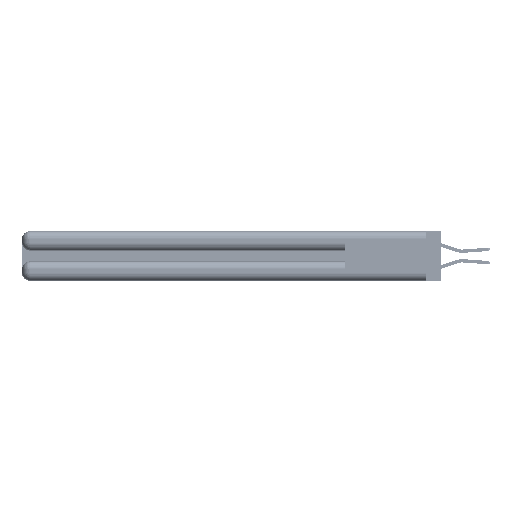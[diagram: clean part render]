
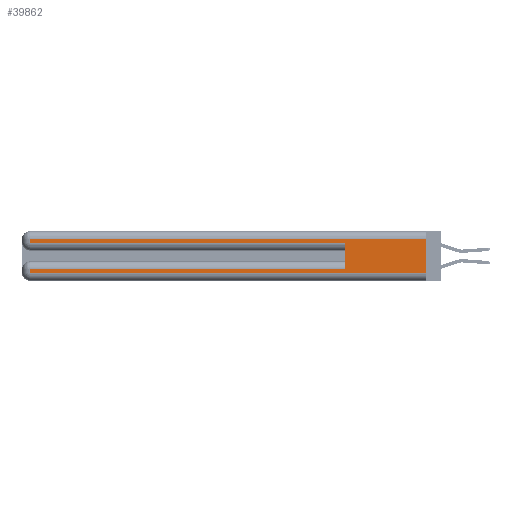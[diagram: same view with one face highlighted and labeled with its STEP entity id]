
A CAD part, left-side view. The second image highlights one B-rep face of the part: STEP entity #39862.
In plain terms, the highlighted planar face has unit normal (-1, 0, 0).
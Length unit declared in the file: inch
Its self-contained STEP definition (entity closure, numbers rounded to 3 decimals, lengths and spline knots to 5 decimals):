
#19 = EDGE_LOOP ( 'NONE', ( #41793, #40045, #23522, #11008, #38077, #45327, #18876, #37443 ) ) ;
#169 = LINE ( 'NONE', #45112, #32521 ) ;
#388 = LINE ( 'NONE', #1569, #31431 ) ;
#1320 = VERTEX_POINT ( 'NONE', #47168 ) ;
#1569 = CARTESIAN_POINT ( 'NONE',  ( 0., 2.94, 0.37 ) ) ;
#1657 = DIRECTION ( 'NONE',  ( 0., 1., 0. ) ) ;
#2510 = CARTESIAN_POINT ( 'NONE',  ( 0., 2.94, 0.285 ) ) ;
#3579 = DIRECTION ( 'NONE',  ( 0., -1., 0. ) ) ;
#3633 = VERTEX_POINT ( 'NONE', #2510 ) ;
#5239 = VECTOR ( 'NONE', #3579, 39.37008 ) ;
#7602 = EDGE_CURVE ( 'NONE', #53940, #32389, #27688, .T. ) ;
#9394 = VECTOR ( 'NONE', #11906, 39.37008 ) ;
#11008 = ORIENTED_EDGE ( 'NONE', *, *, #33853, .T. ) ;
#11906 = DIRECTION ( 'NONE',  ( 0., 0., -1. ) ) ;
#12289 = PLANE ( 'NONE',  #41808 ) ;
#12951 = VERTEX_POINT ( 'NONE', #17623 ) ;
#13339 = CARTESIAN_POINT ( 'NONE',  ( 0., 0., 0.31 ) ) ;
#14971 = CARTESIAN_POINT ( 'NONE',  ( 0., 2.94, 0.31 ) ) ;
#14999 = EDGE_CURVE ( 'NONE', #12951, #39298, #43915, .T. ) ;
#15232 = EDGE_CURVE ( 'NONE', #39298, #53940, #48528, .T. ) ;
#16108 = CARTESIAN_POINT ( 'NONE',  ( 0., 0., 0.06 ) ) ;
#16532 = DIRECTION ( 'NONE',  ( 0., 0., -1. ) ) ;
#17623 = CARTESIAN_POINT ( 'NONE',  ( 0., 0.6, 0.085 ) ) ;
#18876 = ORIENTED_EDGE ( 'NONE', *, *, #15232, .T. ) ;
#21177 = CARTESIAN_POINT ( 'NONE',  ( 0., 0., 0.285 ) ) ;
#22889 = VERTEX_POINT ( 'NONE', #14971 ) ;
#23522 = ORIENTED_EDGE ( 'NONE', *, *, #53543, .T. ) ;
#24090 = DIRECTION ( 'NONE',  ( 0., 0., 1. ) ) ;
#24124 = VECTOR ( 'NONE', #1657, 39.37008 ) ;
#25426 = DIRECTION ( 'NONE',  ( 0., -1., 0. ) ) ;
#26855 = DIRECTION ( 'NONE',  ( 0., 0., -1. ) ) ;
#26941 = CARTESIAN_POINT ( 'NONE',  ( 0., 0., 0.085 ) ) ;
#27688 = LINE ( 'NONE', #16108, #5239 ) ;
#30263 = FACE_OUTER_BOUND ( 'NONE', #19, .T. ) ;
#30709 = EDGE_CURVE ( 'NONE', #12951, #41494, #169, .T. ) ;
#31431 = VECTOR ( 'NONE', #26855, 39.37008 ) ;
#32170 = VECTOR ( 'NONE', #25426, 39.37008 ) ;
#32389 = VERTEX_POINT ( 'NONE', #45517 ) ;
#32521 = VECTOR ( 'NONE', #24090, 39.37008 ) ;
#32956 = CARTESIAN_POINT ( 'NONE',  ( 0., 0., 0.37 ) ) ;
#33336 = VECTOR ( 'NONE', #49042, 39.37008 ) ;
#33473 = LINE ( 'NONE', #21177, #32170 ) ;
#33578 = CARTESIAN_POINT ( 'NONE',  ( 0., 2.94, 0.085 ) ) ;
#33853 = EDGE_CURVE ( 'NONE', #3633, #41494, #33473, .T. ) ;
#37443 = ORIENTED_EDGE ( 'NONE', *, *, #7602, .T. ) ;
#37592 = CARTESIAN_POINT ( 'NONE',  ( 0., 0., 0.37 ) ) ;
#38077 = ORIENTED_EDGE ( 'NONE', *, *, #30709, .F. ) ;
#38658 = DIRECTION ( 'NONE',  ( 0., 1., 0. ) ) ;
#39298 = VERTEX_POINT ( 'NONE', #33578 ) ;
#39862 = ADVANCED_FACE ( 'NONE', ( #30263 ), #12289, .F. ) ;
#40045 = ORIENTED_EDGE ( 'NONE', *, *, #40346, .T. ) ;
#40346 = EDGE_CURVE ( 'NONE', #1320, #22889, #41411, .T. ) ;
#41411 = LINE ( 'NONE', #13339, #51311 ) ;
#41494 = VERTEX_POINT ( 'NONE', #54573 ) ;
#41793 = ORIENTED_EDGE ( 'NONE', *, *, #48043, .F. ) ;
#41808 = AXIS2_PLACEMENT_3D ( 'NONE', #37592, #41818, #16532 ) ;
#41818 = DIRECTION ( 'NONE',  ( 1., 0., 0. ) ) ;
#43043 = LINE ( 'NONE', #32956, #9394 ) ;
#43915 = LINE ( 'NONE', #26941, #24124 ) ;
#45112 = CARTESIAN_POINT ( 'NONE',  ( 0., 0.6, 0.145 ) ) ;
#45327 = ORIENTED_EDGE ( 'NONE', *, *, #14999, .T. ) ;
#45517 = CARTESIAN_POINT ( 'NONE',  ( 0., 0., 0.06 ) ) ;
#47168 = CARTESIAN_POINT ( 'NONE',  ( 0., 0., 0.31 ) ) ;
#48043 = EDGE_CURVE ( 'NONE', #1320, #32389, #43043, .T. ) ;
#48528 = LINE ( 'NONE', #53088, #33336 ) ;
#49042 = DIRECTION ( 'NONE',  ( 0., 0., -1. ) ) ;
#50209 = CARTESIAN_POINT ( 'NONE',  ( 0., 2.94, 0.06 ) ) ;
#51311 = VECTOR ( 'NONE', #38658, 39.37008 ) ;
#53088 = CARTESIAN_POINT ( 'NONE',  ( 0., 2.94, 0.37 ) ) ;
#53543 = EDGE_CURVE ( 'NONE', #22889, #3633, #388, .T. ) ;
#53940 = VERTEX_POINT ( 'NONE', #50209 ) ;
#54573 = CARTESIAN_POINT ( 'NONE',  ( 0., 0.6, 0.285 ) ) ;
